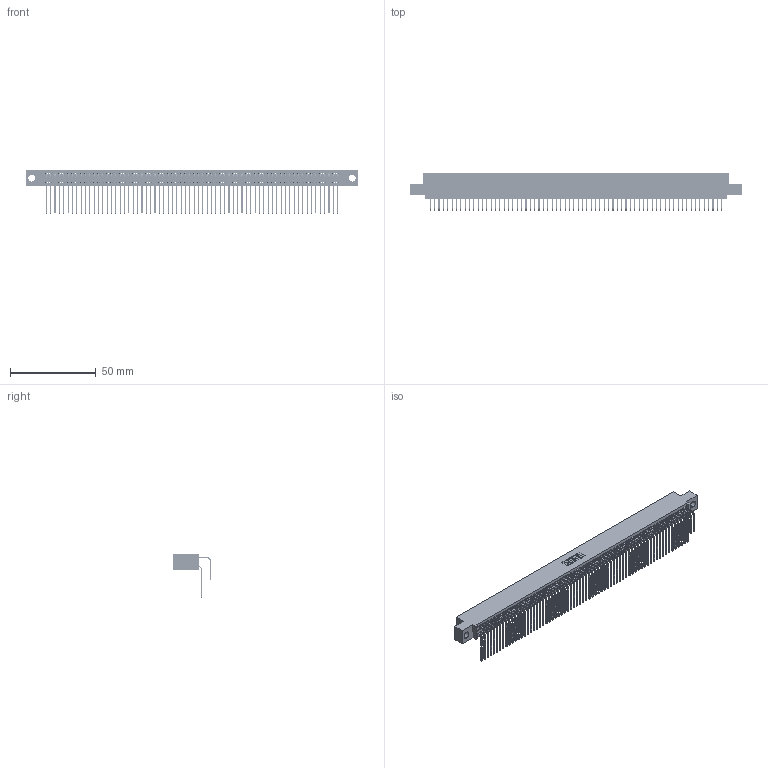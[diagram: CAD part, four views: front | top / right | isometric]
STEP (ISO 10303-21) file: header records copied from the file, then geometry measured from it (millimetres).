
FILE_DESCRIPTION (( 'STEP AP203' ), '1' );
FILE_NAME ('345-136-558-504.STEP', '2021-05-25T23:32:14', ( '' ), ( '' ), 'SwSTEP 2.0', 'SolidWorks 2020', '' );
FILE_SCHEMA (( 'CONFIG_CONTROL_DESIGN' ));
Length unit declared in the file: inch
Products named in the file (4): 345-136-558-504; 345-292-001_558 559 Tail - 1; 345 Part_0.110 Offset - 0.156 Dia-TI; 345-292-001_558 Tail - 2
Assembly tree (137 placements, depth 2):
  345-136-558-504
    345 Part_0.110 Offset - 0.156 Dia-TI
    345-292-001_558 559 Tail - 1  x68
    345-292-001_558 Tail - 2  x68
Bounding box: 193.93 x 21.83 x 25.53 mm (x, y, z)
Volume: 19685 mm3; surface area: 33235 mm2
Topology: 137 solids, 137 shells, 7216 faces, 21469 edges, 14130 vertices
Faces by surface type: plane 4858, cylinder 2358
Entity records: 52057 total; most frequent: CARTESIAN_POINT 8753, ORIENTED_EDGE 8634, DIRECTION 7657, EDGE_CURVE 4317, VECTOR 3873, LINE 3873, VERTEX_POINT 2874, AXIS2_PLACEMENT_3D 1892
